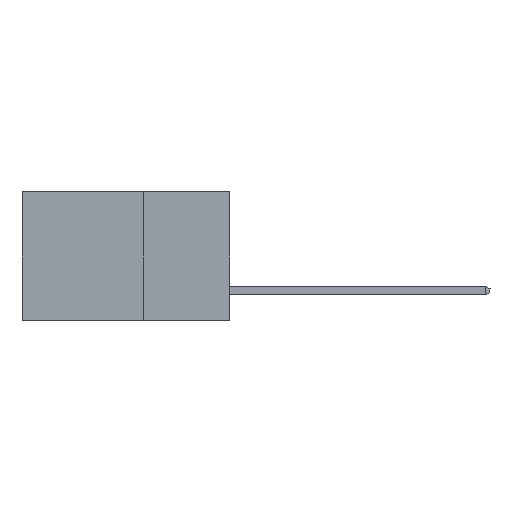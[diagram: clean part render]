
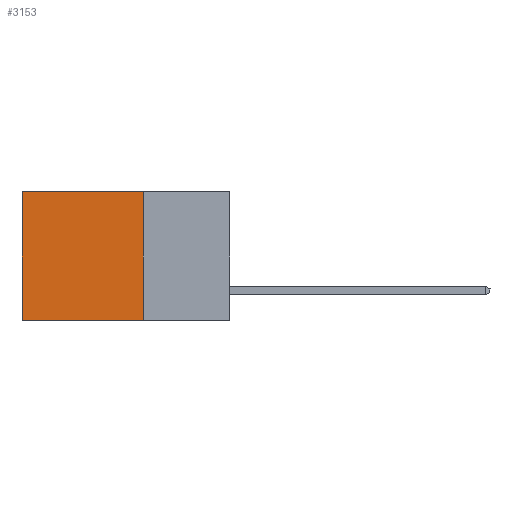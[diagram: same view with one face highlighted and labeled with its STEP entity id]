
A CAD part, left-side view. The second image highlights one B-rep face of the part: STEP entity #3153.
In plain terms, the highlighted planar face has unit normal (-1, 0, 0).
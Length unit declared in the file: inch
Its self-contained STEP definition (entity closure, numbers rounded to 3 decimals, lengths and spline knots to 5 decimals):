
#3 = LINE ( 'NONE', #5361, #20191 ) ;
#800 = LINE ( 'NONE', #4099, #4508 ) ;
#851 = DIRECTION ( 'NONE',  ( 0., 1., 0. ) ) ;
#1256 = CARTESIAN_POINT ( 'NONE',  ( 0.2615, 0.25, -0.37 ) ) ;
#1528 = VECTOR ( 'NONE', #19464, 39.37008 ) ;
#1582 = CARTESIAN_POINT ( 'NONE',  ( 0.2615, 0.25, -0.37 ) ) ;
#1737 = EDGE_CURVE ( 'NONE', #8046, #6673, #800, .T. ) ;
#1836 = EDGE_LOOP ( 'NONE', ( #18610, #21076, #7414, #2108 ) ) ;
#2108 = ORIENTED_EDGE ( 'NONE', *, *, #10074, .T. ) ;
#3153 = ADVANCED_FACE ( 'NONE', ( #12637 ), #4344, .F. ) ;
#4099 = CARTESIAN_POINT ( 'NONE',  ( 0.2615, 0.25, -0.37 ) ) ;
#4307 = VECTOR ( 'NONE', #851, 39.37008 ) ;
#4315 = EDGE_CURVE ( 'NONE', #6673, #20437, #4925, .T. ) ;
#4344 = PLANE ( 'NONE',  #20268 ) ;
#4508 = VECTOR ( 'NONE', #12609, 39.37008 ) ;
#4925 = LINE ( 'NONE', #9962, #1528 ) ;
#5153 = CARTESIAN_POINT ( 'NONE',  ( 0.2615, 0.25, 0. ) ) ;
#5361 = CARTESIAN_POINT ( 'NONE',  ( 0.2615, 0.6, -0.37 ) ) ;
#6673 = VERTEX_POINT ( 'NONE', #1582 ) ;
#7414 = ORIENTED_EDGE ( 'NONE', *, *, #1737, .F. ) ;
#7508 = DIRECTION ( 'NONE',  ( 1., 0., 0. ) ) ;
#8046 = VERTEX_POINT ( 'NONE', #5153 ) ;
#9962 = CARTESIAN_POINT ( 'NONE',  ( 0.2615, 0.25, -0.37 ) ) ;
#10074 = EDGE_CURVE ( 'NONE', #8046, #19430, #11249, .T. ) ;
#11004 = DIRECTION ( 'NONE',  ( 0., 0., -1. ) ) ;
#11249 = LINE ( 'NONE', #17885, #4307 ) ;
#12005 = CARTESIAN_POINT ( 'NONE',  ( 0.2615, 0.6, 0. ) ) ;
#12600 = CARTESIAN_POINT ( 'NONE',  ( 0.2615, 0.6, -0.37 ) ) ;
#12609 = DIRECTION ( 'NONE',  ( 0., 0., -1. ) ) ;
#12637 = FACE_OUTER_BOUND ( 'NONE', #1836, .T. ) ;
#16715 = DIRECTION ( 'NONE',  ( 0., 0., -1. ) ) ;
#17885 = CARTESIAN_POINT ( 'NONE',  ( 0.2615, 0.25, 0. ) ) ;
#18610 = ORIENTED_EDGE ( 'NONE', *, *, #19004, .T. ) ;
#19004 = EDGE_CURVE ( 'NONE', #19430, #20437, #3, .T. ) ;
#19430 = VERTEX_POINT ( 'NONE', #12005 ) ;
#19464 = DIRECTION ( 'NONE',  ( 0., 1., 0. ) ) ;
#20191 = VECTOR ( 'NONE', #16715, 39.37008 ) ;
#20268 = AXIS2_PLACEMENT_3D ( 'NONE', #1256, #7508, #11004 ) ;
#20437 = VERTEX_POINT ( 'NONE', #12600 ) ;
#21076 = ORIENTED_EDGE ( 'NONE', *, *, #4315, .F. ) ;
